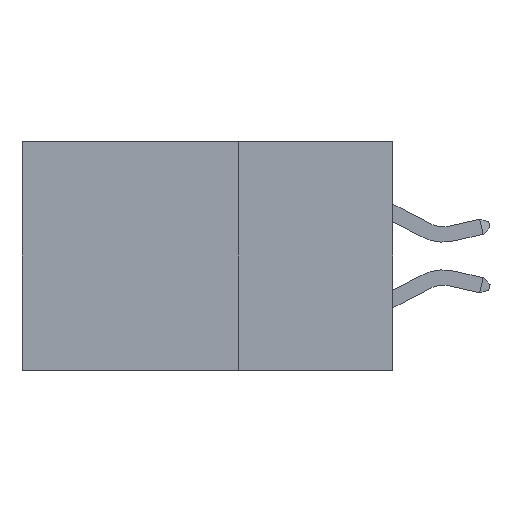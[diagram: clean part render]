
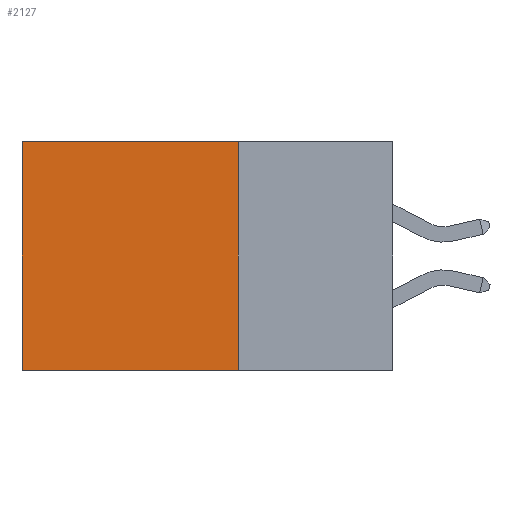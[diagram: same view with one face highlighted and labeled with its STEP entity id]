
A CAD part, left-side view. The second image highlights one B-rep face of the part: STEP entity #2127.
In plain terms, the highlighted planar face has unit normal (-1, 0, 0).
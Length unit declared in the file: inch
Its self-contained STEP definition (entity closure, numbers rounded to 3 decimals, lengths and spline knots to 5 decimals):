
#554 = CARTESIAN_POINT ( 'NONE',  ( 0.2875, 0.25, 0. ) ) ;
#767 = CARTESIAN_POINT ( 'NONE',  ( 0.2875, 0.6, -0.37 ) ) ;
#769 = EDGE_CURVE ( 'NONE', #7840, #19410, #21286, .T. ) ;
#2127 = ADVANCED_FACE ( 'NONE', ( #7296 ), #18742, .F. ) ;
#2326 = ORIENTED_EDGE ( 'NONE', *, *, #16227, .T. ) ;
#3737 = ORIENTED_EDGE ( 'NONE', *, *, #5712, .F. ) ;
#5712 = EDGE_CURVE ( 'NONE', #14696, #6659, #21868, .T. ) ;
#6107 = VECTOR ( 'NONE', #10996, 39.37008 ) ;
#6659 = VERTEX_POINT ( 'NONE', #767 ) ;
#6669 = CARTESIAN_POINT ( 'NONE',  ( 0.2875, 0.25, -0.37 ) ) ;
#7296 = FACE_OUTER_BOUND ( 'NONE', #12610, .T. ) ;
#7305 = CARTESIAN_POINT ( 'NONE',  ( 0.2875, 0.25, 0. ) ) ;
#7840 = VERTEX_POINT ( 'NONE', #554 ) ;
#8520 = DIRECTION ( 'NONE',  ( 1., 0., 0. ) ) ;
#9835 = CARTESIAN_POINT ( 'NONE',  ( 0.2875, 0.25, 0. ) ) ;
#10996 = DIRECTION ( 'NONE',  ( 0., 0., -1. ) ) ;
#12610 = EDGE_LOOP ( 'NONE', ( #2326, #3737, #15346, #14481 ) ) ;
#14440 = VECTOR ( 'NONE', #20800, 39.37008 ) ;
#14481 = ORIENTED_EDGE ( 'NONE', *, *, #769, .T. ) ;
#14696 = VERTEX_POINT ( 'NONE', #6669 ) ;
#15269 = CARTESIAN_POINT ( 'NONE',  ( 0.2875, 0.25, -0.37 ) ) ;
#15282 = EDGE_CURVE ( 'NONE', #7840, #14696, #16851, .T. ) ;
#15346 = ORIENTED_EDGE ( 'NONE', *, *, #15282, .F. ) ;
#16056 = CARTESIAN_POINT ( 'NONE',  ( 0.2875, 0.6, 0. ) ) ;
#16187 = VECTOR ( 'NONE', #19307, 39.37008 ) ;
#16227 = EDGE_CURVE ( 'NONE', #19410, #6659, #19773, .T. ) ;
#16499 = VECTOR ( 'NONE', #20320, 39.37008 ) ;
#16851 = LINE ( 'NONE', #9835, #14440 ) ;
#17075 = CARTESIAN_POINT ( 'NONE',  ( 0.2875, 0.25, 0. ) ) ;
#18260 = AXIS2_PLACEMENT_3D ( 'NONE', #17075, #8520, #20546 ) ;
#18328 = CARTESIAN_POINT ( 'NONE',  ( 0.2875, 0.6, 0. ) ) ;
#18742 = PLANE ( 'NONE',  #18260 ) ;
#19307 = DIRECTION ( 'NONE',  ( 0., 1., 0. ) ) ;
#19410 = VERTEX_POINT ( 'NONE', #18328 ) ;
#19773 = LINE ( 'NONE', #16056, #6107 ) ;
#20320 = DIRECTION ( 'NONE',  ( 0., 1., 0. ) ) ;
#20546 = DIRECTION ( 'NONE',  ( 0., 0., -1. ) ) ;
#20800 = DIRECTION ( 'NONE',  ( 0., 0., -1. ) ) ;
#21286 = LINE ( 'NONE', #7305, #16187 ) ;
#21868 = LINE ( 'NONE', #15269, #16499 ) ;
